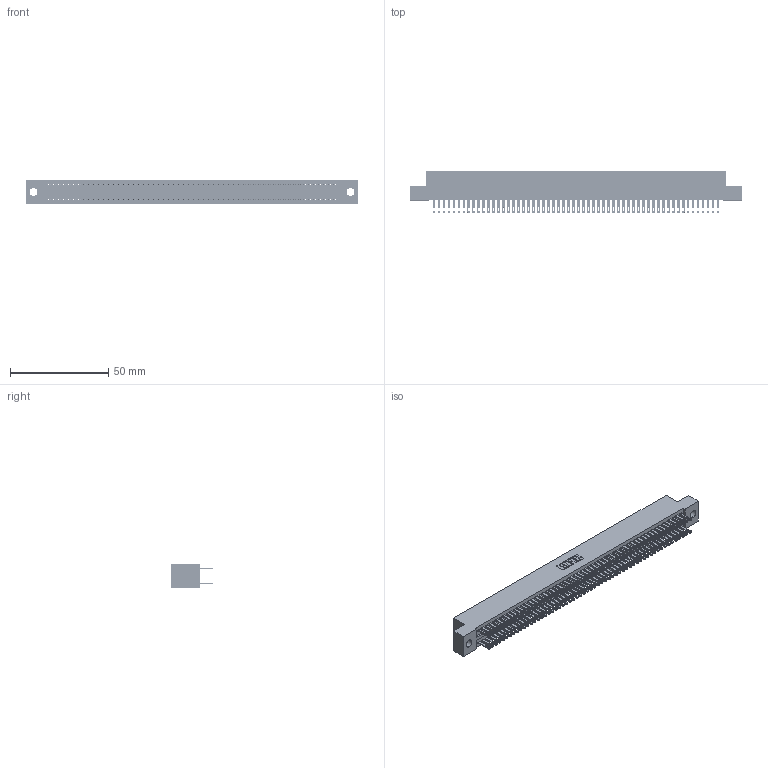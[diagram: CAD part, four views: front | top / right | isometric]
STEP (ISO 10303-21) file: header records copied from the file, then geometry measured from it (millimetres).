
FILE_DESCRIPTION (( 'STEP AP203' ), '1' );
FILE_NAME ('325-116-500-209.STEP', '2020-02-25T08:15:13', ( '' ), ( '' ), 'SwSTEP 2.0', 'SolidWorks 2016', '' );
FILE_SCHEMA (( 'CONFIG_CONTROL_DESIGN' ));
Length unit declared in the file: inch
Products named in the file (3): 325-292-001_325-293-100; 325-116-500-209; 325 Part_.160 TH
Assembly tree (117 placements, depth 2):
  325-116-500-209
    325 Part_.160 TH
    325-292-001_325-293-100  x116
Bounding box: 169.04 x 21.84 x 12.45 mm (x, y, z)
Volume: 22089.2 mm3; surface area: 28248.8 mm2
Topology: 117 solids, 117 shells, 5682 faces, 17363 edges, 11574 vertices
Faces by surface type: plane 3550, cylinder 2132
Entity records: 35177 total; most frequent: CARTESIAN_POINT 5810, ORIENTED_EDGE 5746, DIRECTION 4937, EDGE_CURVE 2873, VECTOR 2741, LINE 2741, VERTEX_POINT 1914, AXIS2_PLACEMENT_3D 1098
